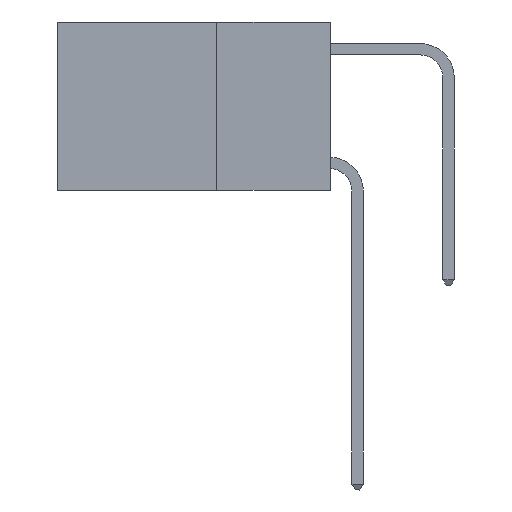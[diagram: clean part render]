
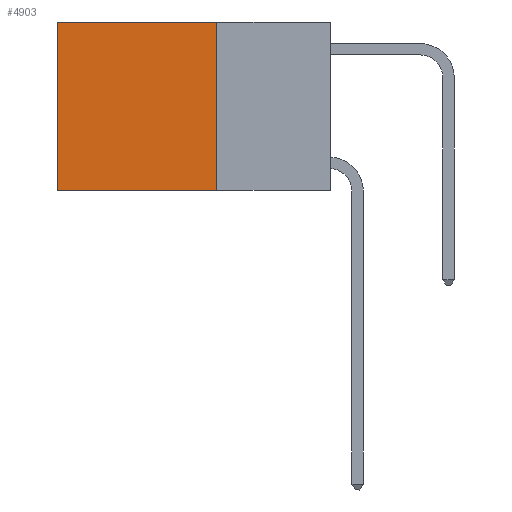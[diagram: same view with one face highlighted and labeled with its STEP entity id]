
A CAD part, left-side view. The second image highlights one B-rep face of the part: STEP entity #4903.
In plain terms, the highlighted planar face has unit normal (-1, 0, 0).
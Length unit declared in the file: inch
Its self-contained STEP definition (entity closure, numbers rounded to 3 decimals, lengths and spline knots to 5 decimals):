
#19 = LINE ( 'NONE', #11153, #2458 ) ;
#59 = ORIENTED_EDGE ( 'NONE', *, *, #5656, .T. ) ;
#2458 = VECTOR ( 'NONE', #5772, 39.37008 ) ;
#2672 = VECTOR ( 'NONE', #12382, 39.37008 ) ;
#3171 = VECTOR ( 'NONE', #14306, 39.37008 ) ;
#3368 = EDGE_CURVE ( 'NONE', #9012, #11454, #19, .T. ) ;
#3459 = ORIENTED_EDGE ( 'NONE', *, *, #11550, .T. ) ;
#3511 = ORIENTED_EDGE ( 'NONE', *, *, #3368, .F. ) ;
#4057 = CARTESIAN_POINT ( 'NONE',  ( 0.2625, 0.6, 0. ) ) ;
#4903 = ADVANCED_FACE ( 'NONE', ( #9001 ), #6896, .F. ) ;
#5053 = CARTESIAN_POINT ( 'NONE',  ( 0.2625, 0.25, 0. ) ) ;
#5375 = LINE ( 'NONE', #13092, #3171 ) ;
#5656 = EDGE_CURVE ( 'NONE', #11793, #11008, #9571, .T. ) ;
#5772 = DIRECTION ( 'NONE',  ( 0., 0., -1. ) ) ;
#6007 = EDGE_CURVE ( 'NONE', #11454, #11008, #5375, .T. ) ;
#6158 = DIRECTION ( 'NONE',  ( 0., 0., -1. ) ) ;
#6258 = CARTESIAN_POINT ( 'NONE',  ( 0.2625, 0.6, 0. ) ) ;
#6817 = CARTESIAN_POINT ( 'NONE',  ( 0.2625, 0.25, 0. ) ) ;
#6896 = PLANE ( 'NONE',  #7545 ) ;
#7059 = ORIENTED_EDGE ( 'NONE', *, *, #6007, .F. ) ;
#7085 = LINE ( 'NONE', #9036, #2672 ) ;
#7545 = AXIS2_PLACEMENT_3D ( 'NONE', #6817, #7858, #10227 ) ;
#7606 = CARTESIAN_POINT ( 'NONE',  ( 0.2625, 0.25, -0.37 ) ) ;
#7858 = DIRECTION ( 'NONE',  ( 1., 0., 0. ) ) ;
#7945 = CARTESIAN_POINT ( 'NONE',  ( 0.2625, 0.6, -0.37 ) ) ;
#9001 = FACE_OUTER_BOUND ( 'NONE', #9992, .T. ) ;
#9012 = VERTEX_POINT ( 'NONE', #5053 ) ;
#9036 = CARTESIAN_POINT ( 'NONE',  ( 0.2625, 0.25, 0. ) ) ;
#9536 = VECTOR ( 'NONE', #6158, 39.37008 ) ;
#9571 = LINE ( 'NONE', #4057, #9536 ) ;
#9992 = EDGE_LOOP ( 'NONE', ( #59, #7059, #3511, #3459 ) ) ;
#10227 = DIRECTION ( 'NONE',  ( 0., 0., -1. ) ) ;
#11008 = VERTEX_POINT ( 'NONE', #7945 ) ;
#11153 = CARTESIAN_POINT ( 'NONE',  ( 0.2625, 0.25, 0. ) ) ;
#11454 = VERTEX_POINT ( 'NONE', #7606 ) ;
#11550 = EDGE_CURVE ( 'NONE', #9012, #11793, #7085, .T. ) ;
#11793 = VERTEX_POINT ( 'NONE', #6258 ) ;
#12382 = DIRECTION ( 'NONE',  ( 0., 1., 0. ) ) ;
#13092 = CARTESIAN_POINT ( 'NONE',  ( 0.2625, 0.25, -0.37 ) ) ;
#14306 = DIRECTION ( 'NONE',  ( 0., 1., 0. ) ) ;
